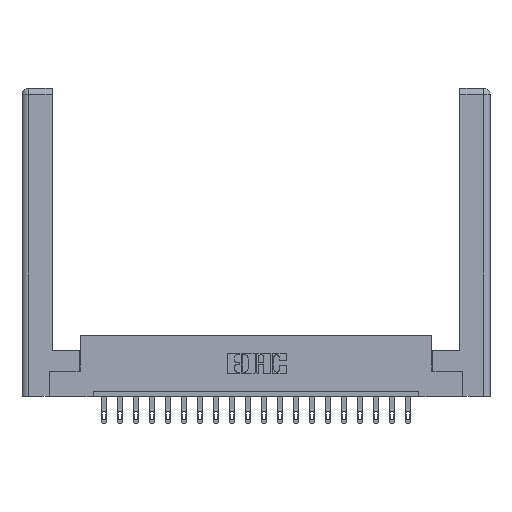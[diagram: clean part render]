
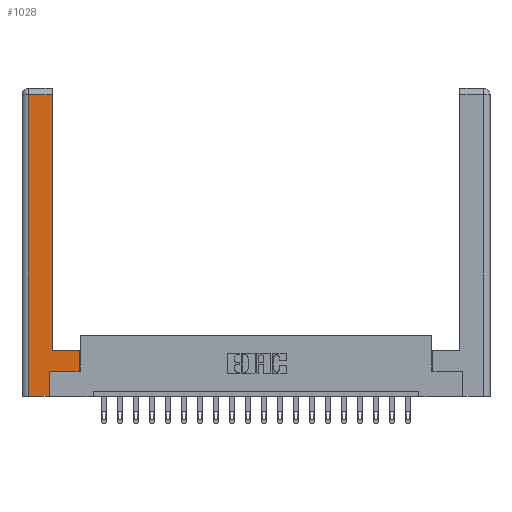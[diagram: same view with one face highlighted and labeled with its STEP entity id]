
A CAD part, top view. The second image highlights one B-rep face of the part: STEP entity #1028.
In plain terms, the highlighted planar face has unit normal (0, 0, 1).
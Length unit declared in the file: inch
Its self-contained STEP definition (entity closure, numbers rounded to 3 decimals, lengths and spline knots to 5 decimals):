
#1028 = ADVANCED_FACE ( 'NONE', ( #19600 ), #16102, .F. ) ;
#1061 = EDGE_CURVE ( 'NONE', #2985, #2963, #15421, .T. ) ;
#1143 = CARTESIAN_POINT ( 'NONE',  ( 0.295, 3., 0. ) ) ;
#1257 = CARTESIAN_POINT ( 'NONE',  ( 0.565, 0.245, 0. ) ) ;
#1283 = ORIENTED_EDGE ( 'NONE', *, *, #16870, .T. ) ;
#1481 = DIRECTION ( 'NONE',  ( 1., 0., 0. ) ) ;
#1525 = VERTEX_POINT ( 'NONE', #13160 ) ;
#1557 = LINE ( 'NONE', #1678, #17768 ) ;
#1678 = CARTESIAN_POINT ( 'NONE',  ( 0.265, 0., 0. ) ) ;
#1916 = VECTOR ( 'NONE', #9596, 39.37008 ) ;
#1926 = VERTEX_POINT ( 'NONE', #13866 ) ;
#2908 = DIRECTION ( 'NONE',  ( 0., 1., 0. ) ) ;
#2963 = VERTEX_POINT ( 'NONE', #1257 ) ;
#2985 = VERTEX_POINT ( 'NONE', #15387 ) ;
#3760 = EDGE_CURVE ( 'NONE', #1525, #1926, #1557, .T. ) ;
#3765 = DIRECTION ( 'NONE',  ( 0., 0., -1. ) ) ;
#3861 = DIRECTION ( 'NONE',  ( 0., 1., 0. ) ) ;
#3998 = VECTOR ( 'NONE', #2908, 39.37008 ) ;
#4200 = VERTEX_POINT ( 'NONE', #9061 ) ;
#4761 = VERTEX_POINT ( 'NONE', #10628 ) ;
#5052 = EDGE_CURVE ( 'NONE', #2963, #4761, #19908, .T. ) ;
#5505 = VECTOR ( 'NONE', #20098, 39.37008 ) ;
#5879 = DIRECTION ( 'NONE',  ( 0., 1., 0. ) ) ;
#5986 = CARTESIAN_POINT ( 'NONE',  ( 0.295, 0.45, 0. ) ) ;
#6347 = VECTOR ( 'NONE', #9923, 39.37008 ) ;
#6682 = LINE ( 'NONE', #1143, #3998 ) ;
#6770 = DIRECTION ( 'NONE',  ( -1., 0., 0. ) ) ;
#6779 = AXIS2_PLACEMENT_3D ( 'NONE', #13158, #3765, #6770 ) ;
#7002 = EDGE_CURVE ( 'NONE', #19093, #1525, #14338, .T. ) ;
#7166 = ORIENTED_EDGE ( 'NONE', *, *, #5052, .T. ) ;
#7573 = CARTESIAN_POINT ( 'NONE',  ( 0.265, 0.245, 0. ) ) ;
#8422 = ORIENTED_EDGE ( 'NONE', *, *, #19461, .T. ) ;
#9061 = CARTESIAN_POINT ( 'NONE',  ( 0.295, 2.94, 0. ) ) ;
#9596 = DIRECTION ( 'NONE',  ( 0., -1., 0. ) ) ;
#9865 = CARTESIAN_POINT ( 'NONE',  ( 0.0615, 0., 0. ) ) ;
#9923 = DIRECTION ( 'NONE',  ( 1., 0., 0. ) ) ;
#9984 = EDGE_LOOP ( 'NONE', ( #12924, #1283, #15207, #10046, #8422, #18385, #7166, #13306 ) ) ;
#10018 = EDGE_CURVE ( 'NONE', #18944, #4200, #6682, .T. ) ;
#10046 = ORIENTED_EDGE ( 'NONE', *, *, #3760, .T. ) ;
#10112 = LINE ( 'NONE', #5986, #14795 ) ;
#10628 = CARTESIAN_POINT ( 'NONE',  ( 0.565, 0.45, 0. ) ) ;
#12924 = ORIENTED_EDGE ( 'NONE', *, *, #10018, .T. ) ;
#13158 = CARTESIAN_POINT ( 'NONE',  ( 0., 0., 0. ) ) ;
#13160 = CARTESIAN_POINT ( 'NONE',  ( 0.0615, 0., 0. ) ) ;
#13306 = ORIENTED_EDGE ( 'NONE', *, *, #14309, .T. ) ;
#13847 = LINE ( 'NONE', #17055, #5505 ) ;
#13866 = CARTESIAN_POINT ( 'NONE',  ( 0.265, 0., 0. ) ) ;
#14034 = VECTOR ( 'NONE', #3861, 39.37008 ) ;
#14309 = EDGE_CURVE ( 'NONE', #4761, #18944, #10112, .T. ) ;
#14338 = LINE ( 'NONE', #9865, #1916 ) ;
#14730 = VECTOR ( 'NONE', #5879, 39.37008 ) ;
#14795 = VECTOR ( 'NONE', #16390, 39.37008 ) ;
#15207 = ORIENTED_EDGE ( 'NONE', *, *, #7002, .T. ) ;
#15387 = CARTESIAN_POINT ( 'NONE',  ( 0.265, 0.245, 0. ) ) ;
#15421 = LINE ( 'NONE', #19321, #6347 ) ;
#16102 = PLANE ( 'NONE',  #6779 ) ;
#16322 = CARTESIAN_POINT ( 'NONE',  ( 0.0615, 2.94, 0. ) ) ;
#16354 = CARTESIAN_POINT ( 'NONE',  ( 0.565, 0.45, 0. ) ) ;
#16390 = DIRECTION ( 'NONE',  ( -1., 0., 0. ) ) ;
#16870 = EDGE_CURVE ( 'NONE', #4200, #19093, #13847, .T. ) ;
#17055 = CARTESIAN_POINT ( 'NONE',  ( 0.0615, 2.94, 0. ) ) ;
#17768 = VECTOR ( 'NONE', #1481, 39.37008 ) ;
#18385 = ORIENTED_EDGE ( 'NONE', *, *, #1061, .T. ) ;
#18903 = LINE ( 'NONE', #7573, #14730 ) ;
#18944 = VERTEX_POINT ( 'NONE', #18996 ) ;
#18996 = CARTESIAN_POINT ( 'NONE',  ( 0.295, 0.45, 0. ) ) ;
#19093 = VERTEX_POINT ( 'NONE', #16322 ) ;
#19321 = CARTESIAN_POINT ( 'NONE',  ( 0.565, 0.245, 0. ) ) ;
#19461 = EDGE_CURVE ( 'NONE', #1926, #2985, #18903, .T. ) ;
#19600 = FACE_OUTER_BOUND ( 'NONE', #9984, .T. ) ;
#19908 = LINE ( 'NONE', #16354, #14034 ) ;
#20098 = DIRECTION ( 'NONE',  ( -1., 0., 0. ) ) ;
